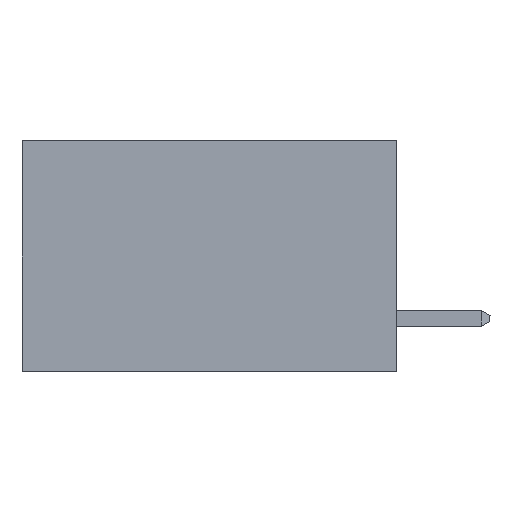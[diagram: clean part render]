
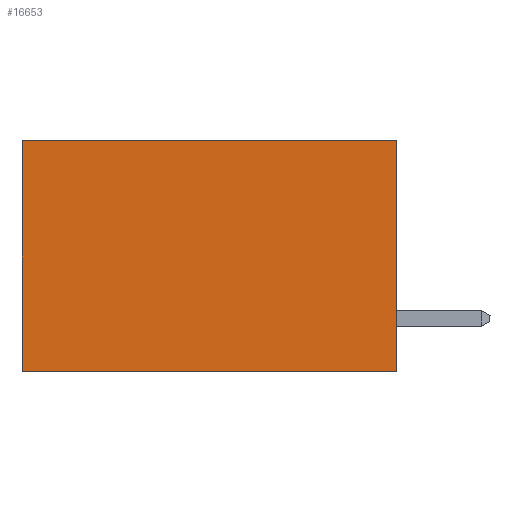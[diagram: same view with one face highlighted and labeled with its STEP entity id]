
A CAD part, left-side view. The second image highlights one B-rep face of the part: STEP entity #16653.
In plain terms, the highlighted planar face has unit normal (-1, 0, 0).
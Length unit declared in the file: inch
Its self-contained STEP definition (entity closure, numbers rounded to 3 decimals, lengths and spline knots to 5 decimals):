
#42 = CARTESIAN_POINT ( 'NONE',  ( 0.2615, 0.6, 0. ) ) ;
#1794 = DIRECTION ( 'NONE',  ( 0., 1., 0. ) ) ;
#2084 = DIRECTION ( 'NONE',  ( 0., 1., 0. ) ) ;
#2272 = VECTOR ( 'NONE', #2084, 39.37008 ) ;
#2741 = CARTESIAN_POINT ( 'NONE',  ( 0.2615, 0., -0.37 ) ) ;
#2933 = EDGE_LOOP ( 'NONE', ( #17503, #9242, #10722, #13961 ) ) ;
#3304 = VECTOR ( 'NONE', #1794, 39.37008 ) ;
#3331 = VERTEX_POINT ( 'NONE', #42 ) ;
#4015 = DIRECTION ( 'NONE',  ( 0., 0., -1. ) ) ;
#5388 = VERTEX_POINT ( 'NONE', #9078 ) ;
#5537 = PLANE ( 'NONE',  #12638 ) ;
#8125 = LINE ( 'NONE', #2741, #15111 ) ;
#8622 = CARTESIAN_POINT ( 'NONE',  ( 0.2615, 0., 0. ) ) ;
#8756 = CARTESIAN_POINT ( 'NONE',  ( 0.2615, 0.6, -0.37 ) ) ;
#9078 = CARTESIAN_POINT ( 'NONE',  ( 0.2615, 0.6, -0.37 ) ) ;
#9242 = ORIENTED_EDGE ( 'NONE', *, *, #16069, .F. ) ;
#10025 = DIRECTION ( 'NONE',  ( 0., 0., -1. ) ) ;
#10236 = VECTOR ( 'NONE', #10025, 39.37008 ) ;
#10722 = ORIENTED_EDGE ( 'NONE', *, *, #12434, .F. ) ;
#11632 = CARTESIAN_POINT ( 'NONE',  ( 0.2615, 0., -0.37 ) ) ;
#11683 = LINE ( 'NONE', #8622, #3304 ) ;
#11751 = EDGE_CURVE ( 'NONE', #13566, #3331, #11683, .T. ) ;
#11938 = CARTESIAN_POINT ( 'NONE',  ( 0.2615, 0., 0. ) ) ;
#12388 = DIRECTION ( 'NONE',  ( 0., 0., -1. ) ) ;
#12407 = CARTESIAN_POINT ( 'NONE',  ( 0.2615, 0., -0.37 ) ) ;
#12434 = EDGE_CURVE ( 'NONE', #13566, #17165, #8125, .T. ) ;
#12605 = EDGE_CURVE ( 'NONE', #3331, #5388, #16735, .T. ) ;
#12638 = AXIS2_PLACEMENT_3D ( 'NONE', #12407, #16575, #4015 ) ;
#13566 = VERTEX_POINT ( 'NONE', #11938 ) ;
#13961 = ORIENTED_EDGE ( 'NONE', *, *, #11751, .T. ) ;
#14401 = LINE ( 'NONE', #11632, #2272 ) ;
#15111 = VECTOR ( 'NONE', #12388, 39.37008 ) ;
#15408 = CARTESIAN_POINT ( 'NONE',  ( 0.2615, 0., -0.37 ) ) ;
#16069 = EDGE_CURVE ( 'NONE', #17165, #5388, #14401, .T. ) ;
#16321 = FACE_OUTER_BOUND ( 'NONE', #2933, .T. ) ;
#16575 = DIRECTION ( 'NONE',  ( 1., 0., 0. ) ) ;
#16653 = ADVANCED_FACE ( 'NONE', ( #16321 ), #5537, .F. ) ;
#16735 = LINE ( 'NONE', #8756, #10236 ) ;
#17165 = VERTEX_POINT ( 'NONE', #15408 ) ;
#17503 = ORIENTED_EDGE ( 'NONE', *, *, #12605, .T. ) ;
